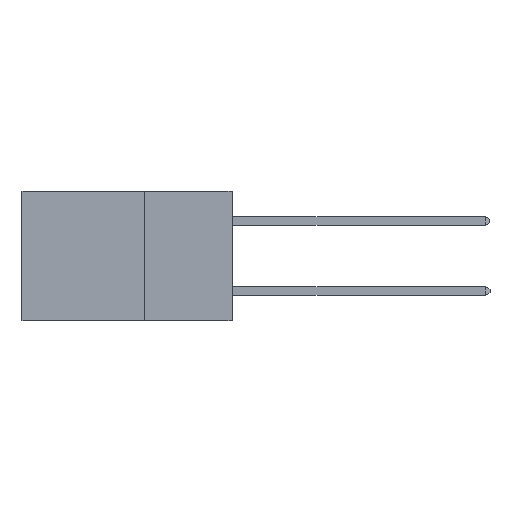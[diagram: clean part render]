
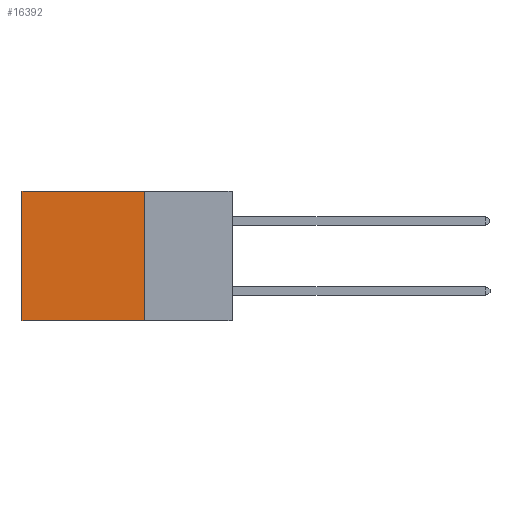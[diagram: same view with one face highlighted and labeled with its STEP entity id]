
A CAD part, left-side view. The second image highlights one B-rep face of the part: STEP entity #16392.
In plain terms, the highlighted planar face has unit normal (-1, 0, 0).
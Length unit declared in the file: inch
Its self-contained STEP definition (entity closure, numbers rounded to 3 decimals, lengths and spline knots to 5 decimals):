
#357 = ORIENTED_EDGE ( 'NONE', *, *, #7599, .T. ) ;
#1121 = CARTESIAN_POINT ( 'NONE',  ( 0.2875, 0.25, 0. ) ) ;
#1327 = DIRECTION ( 'NONE',  ( 0., 0., -1. ) ) ;
#1624 = LINE ( 'NONE', #16156, #12631 ) ;
#1743 = VECTOR ( 'NONE', #1327, 39.37008 ) ;
#4143 = EDGE_CURVE ( 'NONE', #5506, #12050, #1624, .T. ) ;
#4339 = PLANE ( 'NONE',  #17809 ) ;
#4755 = EDGE_LOOP ( 'NONE', ( #12062, #18174, #10550, #357 ) ) ;
#4895 = CARTESIAN_POINT ( 'NONE',  ( 0.2875, 0.25, -0.37 ) ) ;
#5070 = VERTEX_POINT ( 'NONE', #8732 ) ;
#5191 = DIRECTION ( 'NONE',  ( 0., 1., 0. ) ) ;
#5506 = VERTEX_POINT ( 'NONE', #6620 ) ;
#5917 = DIRECTION ( 'NONE',  ( 0., 0., -1. ) ) ;
#6297 = VERTEX_POINT ( 'NONE', #11778 ) ;
#6620 = CARTESIAN_POINT ( 'NONE',  ( 0.2875, 0.25, 0. ) ) ;
#7599 = EDGE_CURVE ( 'NONE', #5506, #6297, #10736, .T. ) ;
#8148 = DIRECTION ( 'NONE',  ( 0., 0., -1. ) ) ;
#8732 = CARTESIAN_POINT ( 'NONE',  ( 0.2875, 0.6, -0.37 ) ) ;
#9913 = CARTESIAN_POINT ( 'NONE',  ( 0.2875, 0.25, -0.37 ) ) ;
#10218 = VECTOR ( 'NONE', #15335, 39.37008 ) ;
#10550 = ORIENTED_EDGE ( 'NONE', *, *, #4143, .F. ) ;
#10736 = LINE ( 'NONE', #20018, #10218 ) ;
#11778 = CARTESIAN_POINT ( 'NONE',  ( 0.2875, 0.6, 0. ) ) ;
#12050 = VERTEX_POINT ( 'NONE', #4895 ) ;
#12062 = ORIENTED_EDGE ( 'NONE', *, *, #19099, .T. ) ;
#12631 = VECTOR ( 'NONE', #8148, 39.37008 ) ;
#13361 = FACE_OUTER_BOUND ( 'NONE', #4755, .T. ) ;
#13651 = VECTOR ( 'NONE', #5191, 39.37008 ) ;
#14512 = LINE ( 'NONE', #20394, #1743 ) ;
#15067 = EDGE_CURVE ( 'NONE', #12050, #5070, #17905, .T. ) ;
#15335 = DIRECTION ( 'NONE',  ( 0., 1., 0. ) ) ;
#15517 = DIRECTION ( 'NONE',  ( 1., 0., 0. ) ) ;
#16156 = CARTESIAN_POINT ( 'NONE',  ( 0.2875, 0.25, 0. ) ) ;
#16392 = ADVANCED_FACE ( 'NONE', ( #13361 ), #4339, .F. ) ;
#17809 = AXIS2_PLACEMENT_3D ( 'NONE', #1121, #15517, #5917 ) ;
#17905 = LINE ( 'NONE', #9913, #13651 ) ;
#18174 = ORIENTED_EDGE ( 'NONE', *, *, #15067, .F. ) ;
#19099 = EDGE_CURVE ( 'NONE', #6297, #5070, #14512, .T. ) ;
#20018 = CARTESIAN_POINT ( 'NONE',  ( 0.2875, 0.25, 0. ) ) ;
#20394 = CARTESIAN_POINT ( 'NONE',  ( 0.2875, 0.6, 0. ) ) ;
